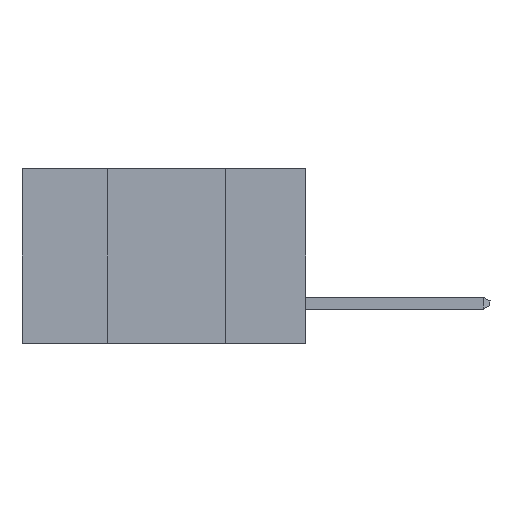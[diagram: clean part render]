
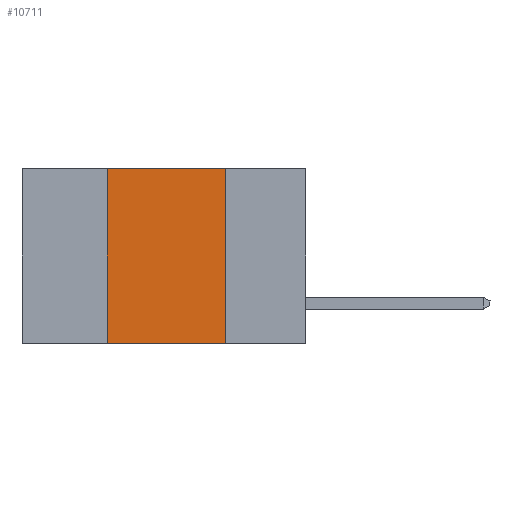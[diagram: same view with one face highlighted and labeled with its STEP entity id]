
A CAD part, left-side view. The second image highlights one B-rep face of the part: STEP entity #10711.
In plain terms, the highlighted planar face has unit normal (-1, 0, 0).
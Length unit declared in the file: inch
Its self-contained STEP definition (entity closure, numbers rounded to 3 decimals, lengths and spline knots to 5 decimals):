
#481 = ORIENTED_EDGE ( 'NONE', *, *, #6403, .F. ) ;
#563 = VECTOR ( 'NONE', #12955, 39.37008 ) ;
#1795 = DIRECTION ( 'NONE',  ( 0., -1., 0. ) ) ;
#1797 = LINE ( 'NONE', #3686, #4239 ) ;
#2119 = EDGE_LOOP ( 'NONE', ( #10190, #4662, #481, #4949 ) ) ;
#3334 = VECTOR ( 'NONE', #8468, 39.37008 ) ;
#3673 = CARTESIAN_POINT ( 'NONE',  ( 0., 0.17, -0.37 ) ) ;
#3686 = CARTESIAN_POINT ( 'NONE',  ( 0., 0.6, 0. ) ) ;
#4239 = VECTOR ( 'NONE', #1795, 39.37008 ) ;
#4662 = ORIENTED_EDGE ( 'NONE', *, *, #12715, .F. ) ;
#4833 = AXIS2_PLACEMENT_3D ( 'NONE', #7950, #7800, #13173 ) ;
#4949 = ORIENTED_EDGE ( 'NONE', *, *, #9248, .T. ) ;
#6289 = LINE ( 'NONE', #8957, #12349 ) ;
#6321 = CARTESIAN_POINT ( 'NONE',  ( 0., 0.42, 0. ) ) ;
#6403 = EDGE_CURVE ( 'NONE', #13246, #11580, #12865, .T. ) ;
#6824 = DIRECTION ( 'NONE',  ( 0., -1., 0. ) ) ;
#6904 = VERTEX_POINT ( 'NONE', #3673 ) ;
#7800 = DIRECTION ( 'NONE',  ( 1., 0., 0. ) ) ;
#7950 = CARTESIAN_POINT ( 'NONE',  ( 0., 0.6, 0. ) ) ;
#8468 = DIRECTION ( 'NONE',  ( 0., 0., -1. ) ) ;
#8747 = CARTESIAN_POINT ( 'NONE',  ( 0., 0.42, 0. ) ) ;
#8800 = VERTEX_POINT ( 'NONE', #13082 ) ;
#8839 = LINE ( 'NONE', #12559, #3334 ) ;
#8957 = CARTESIAN_POINT ( 'NONE',  ( 0., 0.6, -0.37 ) ) ;
#9248 = EDGE_CURVE ( 'NONE', #13246, #6904, #6289, .T. ) ;
#10190 = ORIENTED_EDGE ( 'NONE', *, *, #10803, .F. ) ;
#10711 = ADVANCED_FACE ( 'NONE', ( #12133 ), #11040, .F. ) ;
#10803 = EDGE_CURVE ( 'NONE', #8800, #6904, #8839, .T. ) ;
#10837 = CARTESIAN_POINT ( 'NONE',  ( 0., 0.42, -0.37 ) ) ;
#11040 = PLANE ( 'NONE',  #4833 ) ;
#11580 = VERTEX_POINT ( 'NONE', #6321 ) ;
#12133 = FACE_OUTER_BOUND ( 'NONE', #2119, .T. ) ;
#12349 = VECTOR ( 'NONE', #6824, 39.37008 ) ;
#12559 = CARTESIAN_POINT ( 'NONE',  ( 0., 0.17, 0. ) ) ;
#12715 = EDGE_CURVE ( 'NONE', #11580, #8800, #1797, .T. ) ;
#12865 = LINE ( 'NONE', #8747, #563 ) ;
#12955 = DIRECTION ( 'NONE',  ( 0., 0., 1. ) ) ;
#13082 = CARTESIAN_POINT ( 'NONE',  ( 0., 0.17, 0. ) ) ;
#13173 = DIRECTION ( 'NONE',  ( 0., 0., -1. ) ) ;
#13246 = VERTEX_POINT ( 'NONE', #10837 ) ;
